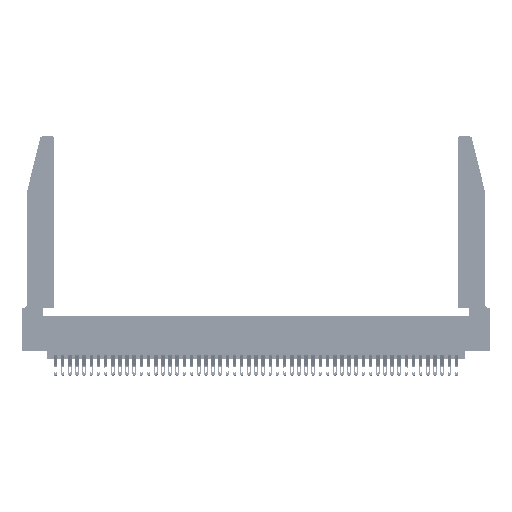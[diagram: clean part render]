
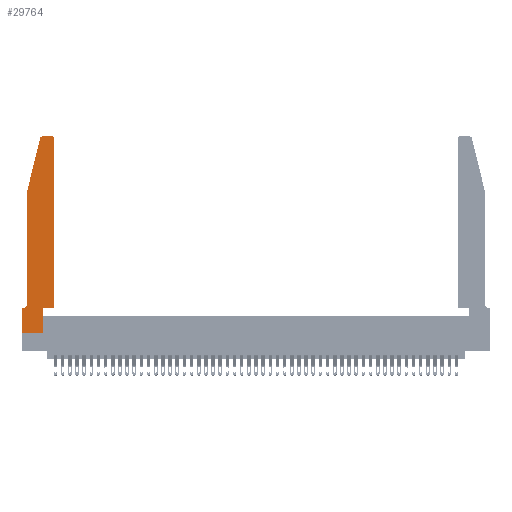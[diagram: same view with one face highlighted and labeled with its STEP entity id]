
A CAD part, top view. The second image highlights one B-rep face of the part: STEP entity #29764.
In plain terms, the highlighted planar face has unit normal (0, 0, 1).
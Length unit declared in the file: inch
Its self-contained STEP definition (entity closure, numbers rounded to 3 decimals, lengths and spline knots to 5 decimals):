
#1054 = CARTESIAN_POINT ( 'NONE',  ( 0.4505, 2.72, 0.37 ) ) ;
#1383 = EDGE_CURVE ( 'NONE', #12450, #19191, #14865, .T. ) ;
#1599 = VECTOR ( 'NONE', #35593, 39.37008 ) ;
#1953 = VECTOR ( 'NONE', #2331, 39.37008 ) ;
#2331 = DIRECTION ( 'NONE',  ( 0., -1., 0. ) ) ;
#3064 = VERTEX_POINT ( 'NONE', #1054 ) ;
#3383 = EDGE_CURVE ( 'NONE', #17929, #45169, #16459, .T. ) ;
#3641 = VERTEX_POINT ( 'NONE', #3762 ) ;
#3658 = ORIENTED_EDGE ( 'NONE', *, *, #4746, .T. ) ;
#3762 = CARTESIAN_POINT ( 'NONE',  ( 0.0755, 0.42, 0.37 ) ) ;
#3828 = DIRECTION ( 'NONE',  ( 1., 0., 0. ) ) ;
#3859 = CARTESIAN_POINT ( 'NONE',  ( 0.2865, 0., 0.37 ) ) ;
#4379 = ORIENTED_EDGE ( 'NONE', *, *, #1383, .T. ) ;
#4706 = EDGE_CURVE ( 'NONE', #19191, #23047, #33193, .T. ) ;
#4746 = EDGE_CURVE ( 'NONE', #45820, #3641, #43581, .T. ) ;
#4999 = VECTOR ( 'NONE', #7728, 39.37008 ) ;
#6125 = DIRECTION ( 'NONE',  ( 0., 0., 1. ) ) ;
#6680 = CARTESIAN_POINT ( 'NONE',  ( 0.0755, 2., 0.37 ) ) ;
#7549 = DIRECTION ( 'NONE',  ( 0., -1., 0. ) ) ;
#7728 = DIRECTION ( 'NONE',  ( 0., 1., 0. ) ) ;
#7954 = LINE ( 'NONE', #31722, #1599 ) ;
#8179 = AXIS2_PLACEMENT_3D ( 'NONE', #34889, #8346, #12367 ) ;
#8346 = DIRECTION ( 'NONE',  ( 0., 0., 1. ) ) ;
#8803 = AXIS2_PLACEMENT_3D ( 'NONE', #26648, #30865, #16260 ) ;
#10006 = CARTESIAN_POINT ( 'NONE',  ( 0.284, 2.72, 0.37 ) ) ;
#12367 = DIRECTION ( 'NONE',  ( 1., 0., 0. ) ) ;
#12450 = VERTEX_POINT ( 'NONE', #3859 ) ;
#12766 = CIRCLE ( 'NONE', #19908, 0.07 ) ;
#13033 = EDGE_CURVE ( 'NONE', #24319, #47796, #14686, .T. ) ;
#13292 = DIRECTION ( 'NONE',  ( -1., 0., 0. ) ) ;
#13543 = CARTESIAN_POINT ( 'NONE',  ( 0., 0., 0.37 ) ) ;
#13696 = DIRECTION ( 'NONE',  ( 1., 0., 0. ) ) ;
#13930 = VERTEX_POINT ( 'NONE', #33735 ) ;
#14686 = LINE ( 'NONE', #36520, #18196 ) ;
#14865 = LINE ( 'NONE', #44663, #4999 ) ;
#14932 = AXIS2_PLACEMENT_3D ( 'NONE', #10006, #6125, #28044 ) ;
#15069 = LINE ( 'NONE', #35589, #21460 ) ;
#15260 = CARTESIAN_POINT ( 'NONE',  ( 0.2865, 0.35, 0.37 ) ) ;
#16260 = DIRECTION ( 'NONE',  ( 1., 0., 0. ) ) ;
#16335 = CARTESIAN_POINT ( 'NONE',  ( 0.25487, 2.72718, 0.37 ) ) ;
#16459 = LINE ( 'NONE', #17549, #1953 ) ;
#17549 = CARTESIAN_POINT ( 'NONE',  ( 0., 0., 0.37 ) ) ;
#17558 = EDGE_CURVE ( 'NONE', #23047, #3064, #38494, .T. ) ;
#17929 = VERTEX_POINT ( 'NONE', #25562 ) ;
#18196 = VECTOR ( 'NONE', #43627, 39.37008 ) ;
#18441 = ORIENTED_EDGE ( 'NONE', *, *, #36703, .T. ) ;
#19191 = VERTEX_POINT ( 'NONE', #15260 ) ;
#19908 = AXIS2_PLACEMENT_3D ( 'NONE', #43082, #20934, #13292 ) ;
#20145 = EDGE_CURVE ( 'NONE', #45169, #12450, #15069, .T. ) ;
#20934 = DIRECTION ( 'NONE',  ( 0., 0., -1. ) ) ;
#21460 = VECTOR ( 'NONE', #13696, 39.37008 ) ;
#23047 = VERTEX_POINT ( 'NONE', #28095 ) ;
#23381 = PLANE ( 'NONE',  #8803 ) ;
#24319 = VERTEX_POINT ( 'NONE', #29302 ) ;
#24341 = VECTOR ( 'NONE', #27564, 39.37008 ) ;
#24828 = EDGE_LOOP ( 'NONE', ( #28317, #25412, #28745, #3658, #18441, #37110, #25117, #39637, #4379, #43364, #30247, #39703 ) ) ;
#25117 = ORIENTED_EDGE ( 'NONE', *, *, #3383, .T. ) ;
#25412 = ORIENTED_EDGE ( 'NONE', *, *, #26080, .T. ) ;
#25562 = CARTESIAN_POINT ( 'NONE',  ( 0., 0.35, 0.37 ) ) ;
#26080 = EDGE_CURVE ( 'NONE', #47796, #39404, #35623, .T. ) ;
#26648 = CARTESIAN_POINT ( 'NONE',  ( 0., 0.35, 0.37 ) ) ;
#27564 = DIRECTION ( 'NONE',  ( 0., 1., 0. ) ) ;
#28044 = DIRECTION ( 'NONE',  ( 1., 0., 0. ) ) ;
#28095 = CARTESIAN_POINT ( 'NONE',  ( 0.4505, 0.35, 0.37 ) ) ;
#28317 = ORIENTED_EDGE ( 'NONE', *, *, #13033, .T. ) ;
#28404 = FACE_OUTER_BOUND ( 'NONE', #24828, .T. ) ;
#28573 = VECTOR ( 'NONE', #7549, 39.37008 ) ;
#28745 = ORIENTED_EDGE ( 'NONE', *, *, #32334, .T. ) ;
#28800 = LINE ( 'NONE', #39891, #37453 ) ;
#29302 = CARTESIAN_POINT ( 'NONE',  ( 0.4205, 2.75, 0.37 ) ) ;
#29453 = CARTESIAN_POINT ( 'NONE',  ( 0.0755, 2., 0.37 ) ) ;
#29764 = ADVANCED_FACE ( 'NONE', ( #28404 ), #23381, .T. ) ;
#30247 = ORIENTED_EDGE ( 'NONE', *, *, #17558, .T. ) ;
#30300 = VECTOR ( 'NONE', #3828, 39.37008 ) ;
#30865 = DIRECTION ( 'NONE',  ( 0., 0., 1. ) ) ;
#31722 = CARTESIAN_POINT ( 'NONE',  ( 0.0755, 2., 0.37 ) ) ;
#32156 = DIRECTION ( 'NONE',  ( -1., 0., 0. ) ) ;
#32334 = EDGE_CURVE ( 'NONE', #39404, #45820, #7954, .T. ) ;
#33193 = LINE ( 'NONE', #47841, #30300 ) ;
#33735 = CARTESIAN_POINT ( 'NONE',  ( 0.0055, 0.35, 0.37 ) ) ;
#34889 = CARTESIAN_POINT ( 'NONE',  ( 0.4205, 2.72, 0.37 ) ) ;
#35589 = CARTESIAN_POINT ( 'NONE',  ( 0., 0., 0.37 ) ) ;
#35593 = DIRECTION ( 'NONE',  ( -0.239, -0.971, 0. ) ) ;
#35623 = CIRCLE ( 'NONE', #14932, 0.03 ) ;
#36520 = CARTESIAN_POINT ( 'NONE',  ( 0.2605, 2.75, 0.37 ) ) ;
#36703 = EDGE_CURVE ( 'NONE', #3641, #13930, #12766, .T. ) ;
#37110 = ORIENTED_EDGE ( 'NONE', *, *, #44567, .T. ) ;
#37453 = VECTOR ( 'NONE', #32156, 39.37008 ) ;
#38494 = LINE ( 'NONE', #38694, #24341 ) ;
#38694 = CARTESIAN_POINT ( 'NONE',  ( 0.4505, 0.35, 0.37 ) ) ;
#39404 = VERTEX_POINT ( 'NONE', #16335 ) ;
#39437 = CARTESIAN_POINT ( 'NONE',  ( 0.284, 2.75, 0.37 ) ) ;
#39637 = ORIENTED_EDGE ( 'NONE', *, *, #20145, .T. ) ;
#39703 = ORIENTED_EDGE ( 'NONE', *, *, #39894, .T. ) ;
#39891 = CARTESIAN_POINT ( 'NONE',  ( 0.0755, 0.35, 0.37 ) ) ;
#39894 = EDGE_CURVE ( 'NONE', #3064, #24319, #40519, .T. ) ;
#40519 = CIRCLE ( 'NONE', #8179, 0.03 ) ;
#43082 = CARTESIAN_POINT ( 'NONE',  ( 0.0055, 0.42, 0.37 ) ) ;
#43364 = ORIENTED_EDGE ( 'NONE', *, *, #4706, .T. ) ;
#43581 = LINE ( 'NONE', #29453, #28573 ) ;
#43627 = DIRECTION ( 'NONE',  ( -1., 0., 0. ) ) ;
#44567 = EDGE_CURVE ( 'NONE', #13930, #17929, #28800, .T. ) ;
#44663 = CARTESIAN_POINT ( 'NONE',  ( 0.2865, 0.35, 0.37 ) ) ;
#45169 = VERTEX_POINT ( 'NONE', #13543 ) ;
#45820 = VERTEX_POINT ( 'NONE', #6680 ) ;
#47796 = VERTEX_POINT ( 'NONE', #39437 ) ;
#47841 = CARTESIAN_POINT ( 'NONE',  ( 0.4505, 0.35, 0.37 ) ) ;
